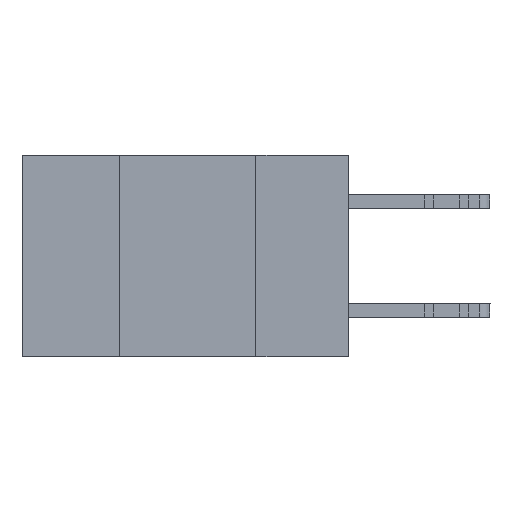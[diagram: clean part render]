
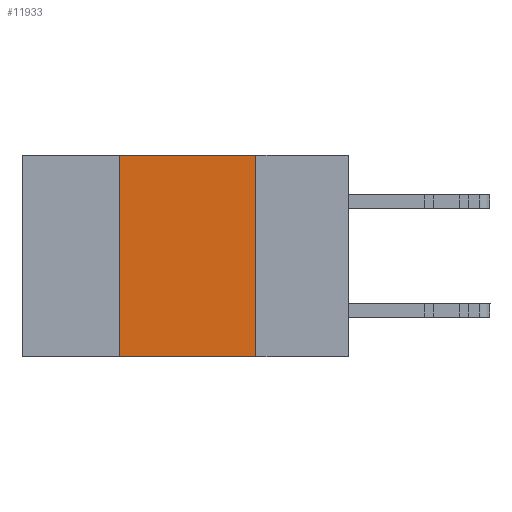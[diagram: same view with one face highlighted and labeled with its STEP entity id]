
A CAD part, left-side view. The second image highlights one B-rep face of the part: STEP entity #11933.
In plain terms, the highlighted planar face has unit normal (-1, 0, 0).
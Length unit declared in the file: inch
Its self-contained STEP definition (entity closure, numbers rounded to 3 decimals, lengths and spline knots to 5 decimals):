
#1576 = CARTESIAN_POINT ( 'NONE',  ( 0., 0.42, -0.37 ) ) ;
#1999 = PLANE ( 'NONE',  #23891 ) ;
#3179 = DIRECTION ( 'NONE',  ( 0., -1., 0. ) ) ;
#3614 = ORIENTED_EDGE ( 'NONE', *, *, #10136, .T. ) ;
#4406 = ORIENTED_EDGE ( 'NONE', *, *, #8862, .F. ) ;
#4838 = CARTESIAN_POINT ( 'NONE',  ( 0., 0.42, -0.37 ) ) ;
#6295 = EDGE_CURVE ( 'NONE', #23911, #21502, #11427, .T. ) ;
#6303 = VERTEX_POINT ( 'NONE', #1576 ) ;
#7092 = DIRECTION ( 'NONE',  ( 0., 0., -1. ) ) ;
#7224 = CARTESIAN_POINT ( 'NONE',  ( 0., 0.17, -0.37 ) ) ;
#7598 = EDGE_CURVE ( 'NONE', #19499, #23911, #18278, .T. ) ;
#8412 = ORIENTED_EDGE ( 'NONE', *, *, #7598, .F. ) ;
#8862 = EDGE_CURVE ( 'NONE', #6303, #19499, #10141, .T. ) ;
#10136 = EDGE_CURVE ( 'NONE', #6303, #21502, #21490, .T. ) ;
#10141 = LINE ( 'NONE', #4838, #14040 ) ;
#11427 = LINE ( 'NONE', #16706, #21043 ) ;
#11580 = DIRECTION ( 'NONE',  ( 0., 0., -1. ) ) ;
#11933 = ADVANCED_FACE ( 'NONE', ( #12978 ), #1999, .F. ) ;
#12699 = CARTESIAN_POINT ( 'NONE',  ( 0., 0.6, 0. ) ) ;
#12978 = FACE_OUTER_BOUND ( 'NONE', #22352, .T. ) ;
#14040 = VECTOR ( 'NONE', #14380, 39.37008 ) ;
#14329 = CARTESIAN_POINT ( 'NONE',  ( 0., 0.6, -0.37 ) ) ;
#14380 = DIRECTION ( 'NONE',  ( 0., 0., 1. ) ) ;
#14737 = ORIENTED_EDGE ( 'NONE', *, *, #6295, .F. ) ;
#16263 = DIRECTION ( 'NONE',  ( 0., -1., 0. ) ) ;
#16395 = VECTOR ( 'NONE', #16263, 39.37008 ) ;
#16706 = CARTESIAN_POINT ( 'NONE',  ( 0., 0.17, -0.37 ) ) ;
#18073 = CARTESIAN_POINT ( 'NONE',  ( 0., 0.17, 0. ) ) ;
#18278 = LINE ( 'NONE', #12699, #20392 ) ;
#19499 = VERTEX_POINT ( 'NONE', #21081 ) ;
#20392 = VECTOR ( 'NONE', #3179, 39.37008 ) ;
#21043 = VECTOR ( 'NONE', #7092, 39.37008 ) ;
#21081 = CARTESIAN_POINT ( 'NONE',  ( 0., 0.42, 0. ) ) ;
#21154 = CARTESIAN_POINT ( 'NONE',  ( 0., 0.6, 0. ) ) ;
#21490 = LINE ( 'NONE', #14329, #16395 ) ;
#21502 = VERTEX_POINT ( 'NONE', #7224 ) ;
#22352 = EDGE_LOOP ( 'NONE', ( #14737, #8412, #4406, #3614 ) ) ;
#23074 = DIRECTION ( 'NONE',  ( 1., 0., 0. ) ) ;
#23891 = AXIS2_PLACEMENT_3D ( 'NONE', #21154, #23074, #11580 ) ;
#23911 = VERTEX_POINT ( 'NONE', #18073 ) ;
